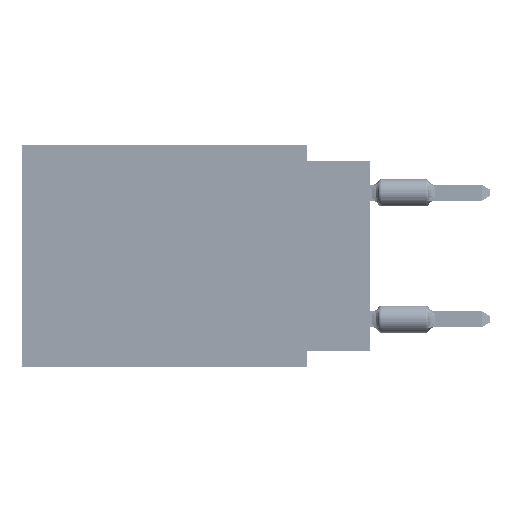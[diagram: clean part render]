
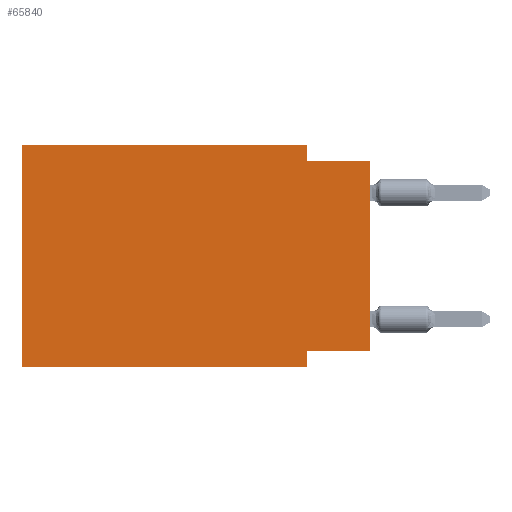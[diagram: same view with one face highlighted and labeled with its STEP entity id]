
A CAD part, left-side view. The second image highlights one B-rep face of the part: STEP entity #65840.
In plain terms, the highlighted planar face has unit normal (-1, 0, 0).
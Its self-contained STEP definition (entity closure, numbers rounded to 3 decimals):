
#1173 = DIRECTION ( 'NONE',  ( 0., 0., -1. ) ) ;
#6653 = ORIENTED_EDGE ( 'NONE', *, *, #71709, .F. ) ;
#7374 = EDGE_CURVE ( 'NONE', #52994, #94645, #59809, .T. ) ;
#7383 = DIRECTION ( 'NONE',  ( 0., 0., 1. ) ) ;
#7995 = VERTEX_POINT ( 'NONE', #49654 ) ;
#9550 = CARTESIAN_POINT ( 'NONE',  ( 0., 0., -0.635 ) ) ;
#11106 = DIRECTION ( 'NONE',  ( 0., 0., -1. ) ) ;
#11673 = CARTESIAN_POINT ( 'NONE',  ( 0., 13.97, 0. ) ) ;
#13430 = VERTEX_POINT ( 'NONE', #83290 ) ;
#13558 = VECTOR ( 'NONE', #98189, 1000. ) ;
#14206 = VECTOR ( 'NONE', #40562, 1000. ) ;
#14491 = DIRECTION ( 'NONE',  ( 0., -1., 0. ) ) ;
#15842 = VECTOR ( 'NONE', #7383, 1000. ) ;
#21275 = VECTOR ( 'NONE', #53189, 1000. ) ;
#25073 = CARTESIAN_POINT ( 'NONE',  ( 0., 13.97, 0. ) ) ;
#27054 = ORIENTED_EDGE ( 'NONE', *, *, #77631, .F. ) ;
#29513 = CARTESIAN_POINT ( 'NONE',  ( 0., 0., -8.255 ) ) ;
#30298 = LINE ( 'NONE', #31760, #15842 ) ;
#31245 = CARTESIAN_POINT ( 'NONE',  ( 0., 13.97, 0. ) ) ;
#31760 = CARTESIAN_POINT ( 'NONE',  ( 0., 0., 0. ) ) ;
#34692 = EDGE_CURVE ( 'NONE', #7995, #49222, #30298, .T. ) ;
#36013 = DIRECTION ( 'NONE',  ( 0., 1., 0. ) ) ;
#36506 = LINE ( 'NONE', #29513, #70270 ) ;
#38199 = CARTESIAN_POINT ( 'NONE',  ( 0., 13.97, 0. ) ) ;
#40562 = DIRECTION ( 'NONE',  ( 0., 0., -1. ) ) ;
#41058 = LINE ( 'NONE', #62995, #14206 ) ;
#43031 = CARTESIAN_POINT ( 'NONE',  ( 0., 2.54, -0.635 ) ) ;
#45360 = LINE ( 'NONE', #82773, #63117 ) ;
#46117 = ORIENTED_EDGE ( 'NONE', *, *, #65969, .F. ) ;
#49222 = VERTEX_POINT ( 'NONE', #9550 ) ;
#49654 = CARTESIAN_POINT ( 'NONE',  ( 0., 0., -8.255 ) ) ;
#50023 = VERTEX_POINT ( 'NONE', #11673 ) ;
#51947 = EDGE_CURVE ( 'NONE', #77766, #49222, #45360, .T. ) ;
#52819 = CARTESIAN_POINT ( 'NONE',  ( 0., 13.97, -8.89 ) ) ;
#52994 = VERTEX_POINT ( 'NONE', #90091 ) ;
#53159 = DIRECTION ( 'NONE',  ( 0., 0., 1. ) ) ;
#53185 = VERTEX_POINT ( 'NONE', #94494 ) ;
#53189 = DIRECTION ( 'NONE',  ( 0., -1., 0. ) ) ;
#53652 = LINE ( 'NONE', #38199, #90805 ) ;
#56568 = CARTESIAN_POINT ( 'NONE',  ( 0., 2.54, -8.89 ) ) ;
#56634 = ORIENTED_EDGE ( 'NONE', *, *, #58204, .F. ) ;
#57038 = VECTOR ( 'NONE', #11106, 1000. ) ;
#58204 = EDGE_CURVE ( 'NONE', #52994, #50023, #53652, .T. ) ;
#59809 = LINE ( 'NONE', #52819, #13558 ) ;
#61459 = FACE_OUTER_BOUND ( 'NONE', #73097, .T. ) ;
#62347 = ORIENTED_EDGE ( 'NONE', *, *, #34692, .T. ) ;
#62995 = CARTESIAN_POINT ( 'NONE',  ( 0., 2.54, -8.89 ) ) ;
#63117 = VECTOR ( 'NONE', #14491, 1000. ) ;
#64349 = ORIENTED_EDGE ( 'NONE', *, *, #83372, .F. ) ;
#64952 = AXIS2_PLACEMENT_3D ( 'NONE', #25073, #76927, #1173 ) ;
#65840 = ADVANCED_FACE ( 'NONE', ( #61459 ), #77920, .F. ) ;
#65969 = EDGE_CURVE ( 'NONE', #13430, #77766, #93851, .T. ) ;
#69643 = LINE ( 'NONE', #31245, #21275 ) ;
#70270 = VECTOR ( 'NONE', #36013, 1000. ) ;
#71709 = EDGE_CURVE ( 'NONE', #7995, #53185, #36506, .T. ) ;
#73097 = EDGE_LOOP ( 'NONE', ( #62347, #83670, #46117, #64349, #56634, #96678, #27054, #6653 ) ) ;
#76927 = DIRECTION ( 'NONE',  ( 1., 0., 0. ) ) ;
#77631 = EDGE_CURVE ( 'NONE', #53185, #94645, #41058, .T. ) ;
#77766 = VERTEX_POINT ( 'NONE', #43031 ) ;
#77920 = PLANE ( 'NONE',  #64952 ) ;
#82773 = CARTESIAN_POINT ( 'NONE',  ( 0., 0., -0.635 ) ) ;
#83290 = CARTESIAN_POINT ( 'NONE',  ( 0., 2.54, 0. ) ) ;
#83372 = EDGE_CURVE ( 'NONE', #50023, #13430, #69643, .T. ) ;
#83670 = ORIENTED_EDGE ( 'NONE', *, *, #51947, .F. ) ;
#90091 = CARTESIAN_POINT ( 'NONE',  ( 0., 13.97, -8.89 ) ) ;
#90805 = VECTOR ( 'NONE', #53159, 1000. ) ;
#93851 = LINE ( 'NONE', #95821, #57038 ) ;
#94494 = CARTESIAN_POINT ( 'NONE',  ( 0., 2.54, -8.255 ) ) ;
#94645 = VERTEX_POINT ( 'NONE', #56568 ) ;
#95821 = CARTESIAN_POINT ( 'NONE',  ( 0., 2.54, 0. ) ) ;
#96678 = ORIENTED_EDGE ( 'NONE', *, *, #7374, .T. ) ;
#98189 = DIRECTION ( 'NONE',  ( 0., -1., 0. ) ) ;
